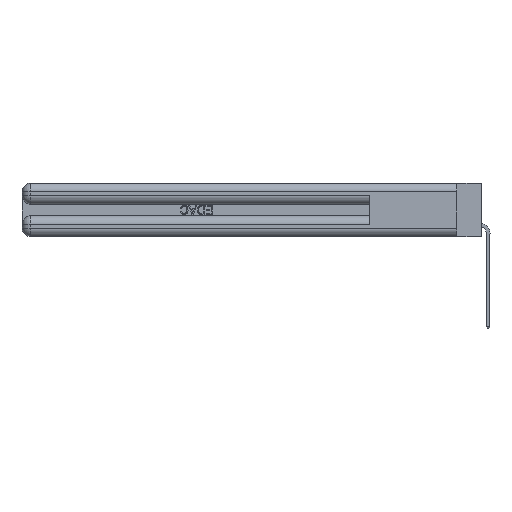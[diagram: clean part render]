
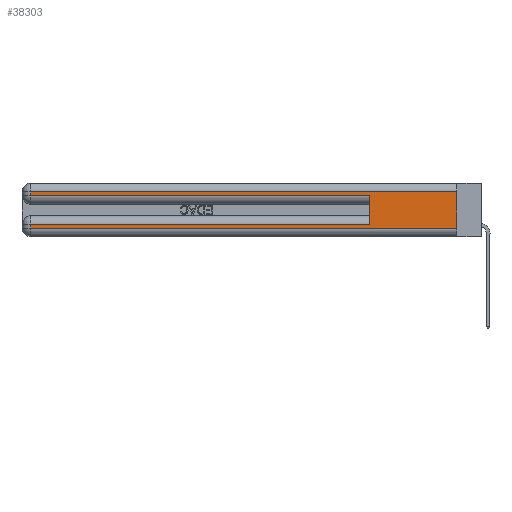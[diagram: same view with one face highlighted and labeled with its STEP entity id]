
A CAD part, left-side view. The second image highlights one B-rep face of the part: STEP entity #38303.
In plain terms, the highlighted planar face has unit normal (-1, 0, 0).
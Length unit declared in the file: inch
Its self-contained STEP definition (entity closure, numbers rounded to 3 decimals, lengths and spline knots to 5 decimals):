
#169 = ORIENTED_EDGE ( 'NONE', *, *, #31814, .F. ) ;
#652 = CARTESIAN_POINT ( 'NONE',  ( 0., 2.94, 0.37 ) ) ;
#1015 = EDGE_CURVE ( 'NONE', #30966, #23986, #16540, .T. ) ;
#2777 = CARTESIAN_POINT ( 'NONE',  ( 0., 0., 0.31 ) ) ;
#4544 = VECTOR ( 'NONE', #23387, 39.37008 ) ;
#4764 = CARTESIAN_POINT ( 'NONE',  ( 0., 0.6, 0.085 ) ) ;
#4808 = ORIENTED_EDGE ( 'NONE', *, *, #27846, .F. ) ;
#5225 = ORIENTED_EDGE ( 'NONE', *, *, #23897, .T. ) ;
#5670 = ORIENTED_EDGE ( 'NONE', *, *, #35363, .T. ) ;
#5778 = DIRECTION ( 'NONE',  ( 1., 0., 0. ) ) ;
#6079 = EDGE_CURVE ( 'NONE', #15529, #12216, #25157, .T. ) ;
#7142 = AXIS2_PLACEMENT_3D ( 'NONE', #20816, #5778, #15172 ) ;
#7345 = DIRECTION ( 'NONE',  ( 0., 1., 0. ) ) ;
#8156 = CARTESIAN_POINT ( 'NONE',  ( 0., 2.94, 0.06 ) ) ;
#9595 = VECTOR ( 'NONE', #32769, 39.37008 ) ;
#9766 = DIRECTION ( 'NONE',  ( 0., 0., -1. ) ) ;
#10955 = VERTEX_POINT ( 'NONE', #32485 ) ;
#11547 = CARTESIAN_POINT ( 'NONE',  ( 0., 0., 0.37 ) ) ;
#12216 = VERTEX_POINT ( 'NONE', #16575 ) ;
#12395 = ORIENTED_EDGE ( 'NONE', *, *, #1015, .T. ) ;
#12540 = ORIENTED_EDGE ( 'NONE', *, *, #6079, .T. ) ;
#12586 = LINE ( 'NONE', #28567, #31645 ) ;
#13114 = CARTESIAN_POINT ( 'NONE',  ( 0., 2.94, 0.37 ) ) ;
#14685 = CARTESIAN_POINT ( 'NONE',  ( 0., 0., 0.31 ) ) ;
#15172 = DIRECTION ( 'NONE',  ( 0., 0., -1. ) ) ;
#15529 = VERTEX_POINT ( 'NONE', #2777 ) ;
#15659 = ORIENTED_EDGE ( 'NONE', *, *, #36686, .T. ) ;
#16540 = LINE ( 'NONE', #29321, #4544 ) ;
#16575 = CARTESIAN_POINT ( 'NONE',  ( 0., 2.94, 0.31 ) ) ;
#17131 = VECTOR ( 'NONE', #7345, 39.37008 ) ;
#17773 = LINE ( 'NONE', #23501, #9595 ) ;
#19200 = LINE ( 'NONE', #652, #21569 ) ;
#20816 = CARTESIAN_POINT ( 'NONE',  ( 0., 0., 0.37 ) ) ;
#21084 = CARTESIAN_POINT ( 'NONE',  ( 0., 2.94, 0.285 ) ) ;
#21569 = VECTOR ( 'NONE', #21781, 39.37008 ) ;
#21700 = LINE ( 'NONE', #11547, #24138 ) ;
#21781 = DIRECTION ( 'NONE',  ( 0., 0., -1. ) ) ;
#23387 = DIRECTION ( 'NONE',  ( 0., 1., 0. ) ) ;
#23501 = CARTESIAN_POINT ( 'NONE',  ( 0., 0., 0.06 ) ) ;
#23897 = EDGE_CURVE ( 'NONE', #12216, #29600, #37470, .T. ) ;
#23986 = VERTEX_POINT ( 'NONE', #25913 ) ;
#24138 = VECTOR ( 'NONE', #29918, 39.37008 ) ;
#24348 = PLANE ( 'NONE',  #7142 ) ;
#25157 = LINE ( 'NONE', #14685, #17131 ) ;
#25913 = CARTESIAN_POINT ( 'NONE',  ( 0., 2.94, 0.085 ) ) ;
#27846 = EDGE_CURVE ( 'NONE', #30966, #10955, #36785, .T. ) ;
#28567 = CARTESIAN_POINT ( 'NONE',  ( 0., 0., 0.285 ) ) ;
#28711 = VECTOR ( 'NONE', #34200, 39.37008 ) ;
#28844 = DIRECTION ( 'NONE',  ( 0., -1., 0. ) ) ;
#29321 = CARTESIAN_POINT ( 'NONE',  ( 0., 0., 0.085 ) ) ;
#29600 = VERTEX_POINT ( 'NONE', #21084 ) ;
#29918 = DIRECTION ( 'NONE',  ( 0., 0., -1. ) ) ;
#30236 = VERTEX_POINT ( 'NONE', #31652 ) ;
#30966 = VERTEX_POINT ( 'NONE', #4764 ) ;
#31645 = VECTOR ( 'NONE', #28844, 39.37008 ) ;
#31652 = CARTESIAN_POINT ( 'NONE',  ( 0., 0., 0.06 ) ) ;
#31814 = EDGE_CURVE ( 'NONE', #15529, #30236, #21700, .T. ) ;
#32320 = VERTEX_POINT ( 'NONE', #8156 ) ;
#32485 = CARTESIAN_POINT ( 'NONE',  ( 0., 0.6, 0.285 ) ) ;
#32769 = DIRECTION ( 'NONE',  ( 0., -1., 0. ) ) ;
#33098 = EDGE_LOOP ( 'NONE', ( #169, #12540, #5225, #5670, #4808, #12395, #37167, #15659 ) ) ;
#34200 = DIRECTION ( 'NONE',  ( 0., 0., 1. ) ) ;
#34848 = FACE_OUTER_BOUND ( 'NONE', #33098, .T. ) ;
#35363 = EDGE_CURVE ( 'NONE', #29600, #10955, #12586, .T. ) ;
#36686 = EDGE_CURVE ( 'NONE', #32320, #30236, #17773, .T. ) ;
#36741 = EDGE_CURVE ( 'NONE', #23986, #32320, #19200, .T. ) ;
#36785 = LINE ( 'NONE', #36989, #28711 ) ;
#36989 = CARTESIAN_POINT ( 'NONE',  ( 0., 0.6, 0.145 ) ) ;
#37167 = ORIENTED_EDGE ( 'NONE', *, *, #36741, .T. ) ;
#37470 = LINE ( 'NONE', #13114, #38474 ) ;
#38303 = ADVANCED_FACE ( 'NONE', ( #34848 ), #24348, .F. ) ;
#38474 = VECTOR ( 'NONE', #9766, 39.37008 ) ;
